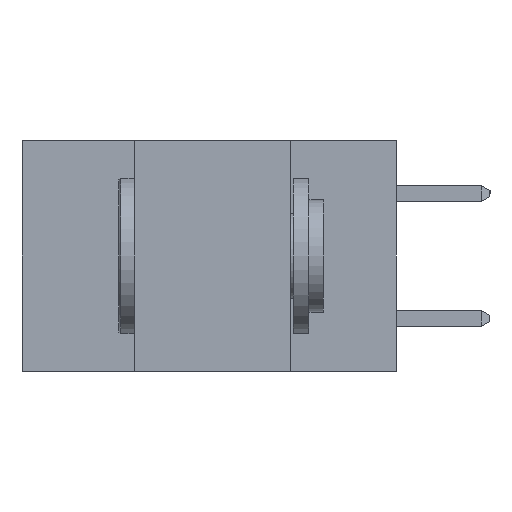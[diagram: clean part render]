
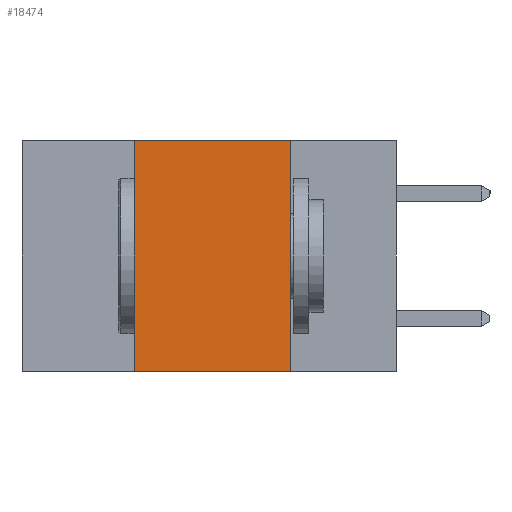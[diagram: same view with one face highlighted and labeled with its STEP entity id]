
A CAD part, left-side view. The second image highlights one B-rep face of the part: STEP entity #18474.
In plain terms, the highlighted planar face has unit normal (-1, 0, 0).
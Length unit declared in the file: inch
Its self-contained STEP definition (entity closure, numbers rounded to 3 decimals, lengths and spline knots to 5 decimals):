
#710 = ORIENTED_EDGE ( 'NONE', *, *, #4629, .F. ) ;
#1567 = ORIENTED_EDGE ( 'NONE', *, *, #20624, .T. ) ;
#2397 = CARTESIAN_POINT ( 'NONE',  ( 0., 0.6, 0. ) ) ;
#2499 = AXIS2_PLACEMENT_3D ( 'NONE', #5949, #17136, #16665 ) ;
#3052 = LINE ( 'NONE', #17892, #17675 ) ;
#4505 = CARTESIAN_POINT ( 'NONE',  ( 0., 0.6, -0.37 ) ) ;
#4588 = EDGE_CURVE ( 'NONE', #22920, #6949, #22280, .T. ) ;
#4629 = EDGE_CURVE ( 'NONE', #14392, #22920, #11592, .T. ) ;
#4643 = VECTOR ( 'NONE', #11480, 39.37008 ) ;
#4817 = ORIENTED_EDGE ( 'NONE', *, *, #8076, .F. ) ;
#4989 = CARTESIAN_POINT ( 'NONE',  ( 0., 0.17, 0. ) ) ;
#5949 = CARTESIAN_POINT ( 'NONE',  ( 0., 0.6, 0. ) ) ;
#6949 = VERTEX_POINT ( 'NONE', #7967 ) ;
#7055 = DIRECTION ( 'NONE',  ( 0., 0., 1. ) ) ;
#7841 = FACE_OUTER_BOUND ( 'NONE', #14855, .T. ) ;
#7967 = CARTESIAN_POINT ( 'NONE',  ( 0., 0.17, -0.37 ) ) ;
#8058 = LINE ( 'NONE', #4505, #22033 ) ;
#8076 = EDGE_CURVE ( 'NONE', #14781, #14392, #3052, .T. ) ;
#11480 = DIRECTION ( 'NONE',  ( 0., -1., 0. ) ) ;
#11592 = LINE ( 'NONE', #2397, #4643 ) ;
#11818 = CARTESIAN_POINT ( 'NONE',  ( 0., 0.17, -0.37 ) ) ;
#14392 = VERTEX_POINT ( 'NONE', #19847 ) ;
#14781 = VERTEX_POINT ( 'NONE', #17470 ) ;
#14855 = EDGE_LOOP ( 'NONE', ( #17375, #710, #4817, #1567 ) ) ;
#14868 = DIRECTION ( 'NONE',  ( 0., -1., 0. ) ) ;
#16665 = DIRECTION ( 'NONE',  ( 0., 0., -1. ) ) ;
#16874 = DIRECTION ( 'NONE',  ( 0., 0., -1. ) ) ;
#17136 = DIRECTION ( 'NONE',  ( 1., 0., 0. ) ) ;
#17375 = ORIENTED_EDGE ( 'NONE', *, *, #4588, .F. ) ;
#17470 = CARTESIAN_POINT ( 'NONE',  ( 0., 0.42, -0.37 ) ) ;
#17675 = VECTOR ( 'NONE', #7055, 39.37008 ) ;
#17892 = CARTESIAN_POINT ( 'NONE',  ( 0., 0.42, -0.37 ) ) ;
#18474 = ADVANCED_FACE ( 'NONE', ( #7841 ), #18685, .F. ) ;
#18685 = PLANE ( 'NONE',  #2499 ) ;
#19847 = CARTESIAN_POINT ( 'NONE',  ( 0., 0.42, 0. ) ) ;
#20624 = EDGE_CURVE ( 'NONE', #14781, #6949, #8058, .T. ) ;
#22033 = VECTOR ( 'NONE', #14868, 39.37008 ) ;
#22280 = LINE ( 'NONE', #11818, #22634 ) ;
#22634 = VECTOR ( 'NONE', #16874, 39.37008 ) ;
#22920 = VERTEX_POINT ( 'NONE', #4989 ) ;
